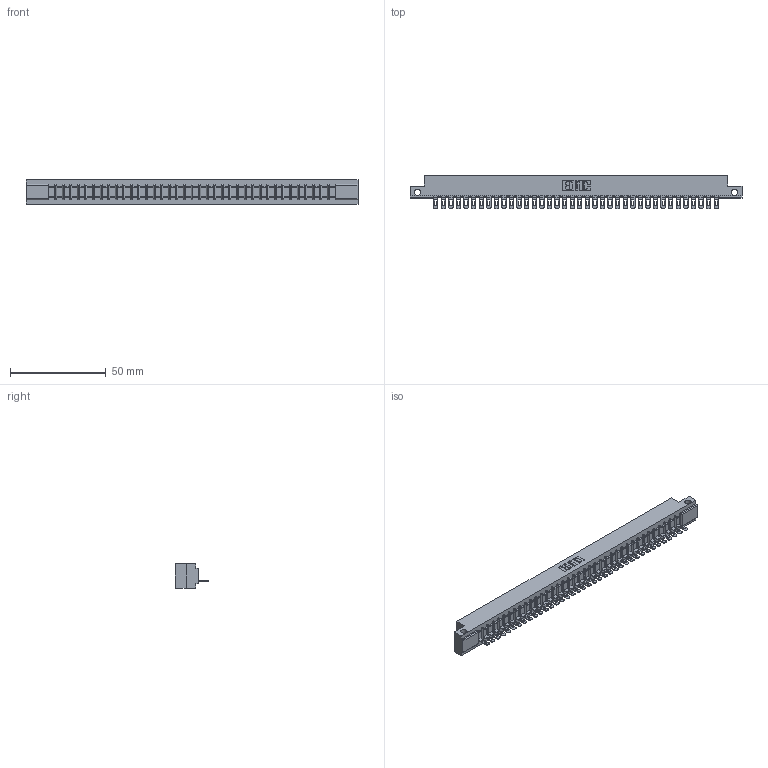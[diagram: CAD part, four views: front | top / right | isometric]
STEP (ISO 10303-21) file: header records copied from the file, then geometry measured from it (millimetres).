
FILE_DESCRIPTION (( 'STEP AP203' ), '1' );
FILE_NAME ('307-038-501-112.STEP', '2018-08-05T11:05:35', ( '' ), ( '' ), 'SwSTEP 2.0', 'SolidWorks 2016', '' );
FILE_SCHEMA (( 'CONFIG_CONTROL_DESIGN' ));
Length unit declared in the file: inch
Products named in the file (3): 307 Part_.128 Dia Side Mounting Holes; 307-290-002_501; 307-038-501-112
Assembly tree (39 placements, depth 2):
  307-038-501-112
    307 Part_.128 Dia Side Mounting Holes
    307-290-002_501  x38
Bounding box: 173.58 x 17.42 x 12.7 mm (x, y, z)
Volume: 18436.8 mm3; surface area: 23339.8 mm2
Topology: 39 solids, 39 shells, 3045 faces, 9367 edges, 6138 vertices
Faces by surface type: plane 1742, cylinder 1225, sphere 78
Entity records: 33866 total; most frequent: CARTESIAN_POINT 5712, ORIENTED_EDGE 5702, DIRECTION 5555, EDGE_CURVE 2851, VECTOR 2177, LINE 2177, VERTEX_POINT 1846, AXIS2_PLACEMENT_3D 1689
